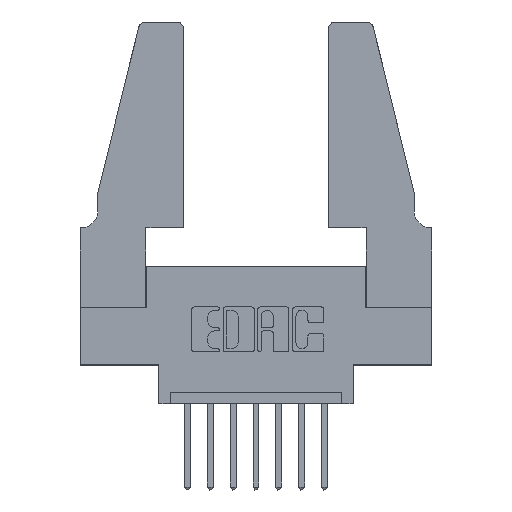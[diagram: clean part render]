
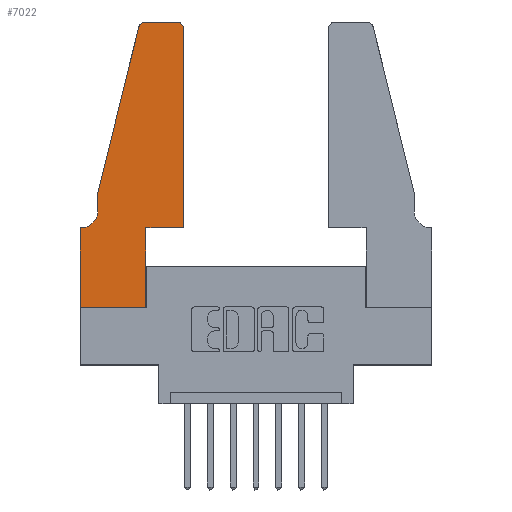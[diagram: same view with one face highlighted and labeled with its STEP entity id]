
A CAD part, top view. The second image highlights one B-rep face of the part: STEP entity #7022.
In plain terms, the highlighted planar face has unit normal (0, 0, 1).
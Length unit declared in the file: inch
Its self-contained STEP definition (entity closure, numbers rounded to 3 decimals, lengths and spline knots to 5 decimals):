
#166 = CARTESIAN_POINT ( 'NONE',  ( 0.0755, 0.42, 0.37 ) ) ;
#304 = LINE ( 'NONE', #4381, #5185 ) ;
#430 = CARTESIAN_POINT ( 'NONE',  ( 0.2865, 0.35, 0.37 ) ) ;
#513 = DIRECTION ( 'NONE',  ( 1., 0., 0. ) ) ;
#522 = LINE ( 'NONE', #9591, #1848 ) ;
#562 = CARTESIAN_POINT ( 'NONE',  ( 0.4505, 0.35, 0.37 ) ) ;
#626 = VECTOR ( 'NONE', #3883, 39.37008 ) ;
#668 = DIRECTION ( 'NONE',  ( 1., 0., 0. ) ) ;
#706 = VECTOR ( 'NONE', #9544, 39.37008 ) ;
#772 = CARTESIAN_POINT ( 'NONE',  ( 0.4205, 1.25, 0.37 ) ) ;
#1071 = VERTEX_POINT ( 'NONE', #3233 ) ;
#1128 = LINE ( 'NONE', #4679, #10800 ) ;
#1173 = CARTESIAN_POINT ( 'NONE',  ( 0.0755, 0.35, 0.37 ) ) ;
#1192 = VERTEX_POINT ( 'NONE', #3646 ) ;
#1230 = ORIENTED_EDGE ( 'NONE', *, *, #9600, .T. ) ;
#1241 = ORIENTED_EDGE ( 'NONE', *, *, #9522, .T. ) ;
#1252 = ORIENTED_EDGE ( 'NONE', *, *, #2379, .T. ) ;
#1300 = EDGE_CURVE ( 'NONE', #8471, #4289, #6045, .T. ) ;
#1409 = VERTEX_POINT ( 'NONE', #11845 ) ;
#1569 = EDGE_CURVE ( 'NONE', #11070, #6706, #1128, .T. ) ;
#1848 = VECTOR ( 'NONE', #3009, 39.37008 ) ;
#2005 = CARTESIAN_POINT ( 'NONE',  ( 0.0755, 0.5, 0.37 ) ) ;
#2217 = PLANE ( 'NONE',  #5233 ) ;
#2340 = CARTESIAN_POINT ( 'NONE',  ( 0., 0.35, 0.37 ) ) ;
#2379 = EDGE_CURVE ( 'NONE', #1192, #2687, #522, .T. ) ;
#2471 = DIRECTION ( 'NONE',  ( 0., 1., 0. ) ) ;
#2560 = EDGE_CURVE ( 'NONE', #1071, #8806, #4241, .T. ) ;
#2619 = DIRECTION ( 'NONE',  ( -0.239, -0.971, 0. ) ) ;
#2687 = VERTEX_POINT ( 'NONE', #9164 ) ;
#3009 = DIRECTION ( 'NONE',  ( 0., -1., 0. ) ) ;
#3233 = CARTESIAN_POINT ( 'NONE',  ( 0.4505, 1.22, 0.37 ) ) ;
#3252 = ORIENTED_EDGE ( 'NONE', *, *, #5866, .T. ) ;
#3311 = LINE ( 'NONE', #7150, #5851 ) ;
#3422 = ORIENTED_EDGE ( 'NONE', *, *, #2560, .T. ) ;
#3570 = DIRECTION ( 'NONE',  ( 0., 0., 1. ) ) ;
#3592 = LINE ( 'NONE', #1173, #626 ) ;
#3646 = CARTESIAN_POINT ( 'NONE',  ( 0., 0.35, 0.37 ) ) ;
#3883 = DIRECTION ( 'NONE',  ( -1., 0., 0. ) ) ;
#4055 = AXIS2_PLACEMENT_3D ( 'NONE', #4297, #11877, #513 ) ;
#4241 = CIRCLE ( 'NONE', #4984, 0.03 ) ;
#4289 = VERTEX_POINT ( 'NONE', #562 ) ;
#4297 = CARTESIAN_POINT ( 'NONE',  ( 0.284, 1.22, 0.37 ) ) ;
#4381 = CARTESIAN_POINT ( 'NONE',  ( 0., 0., 0.37 ) ) ;
#4478 = CARTESIAN_POINT ( 'NONE',  ( 0.0055, 0.35, 0.37 ) ) ;
#4501 = CIRCLE ( 'NONE', #4055, 0.03 ) ;
#4679 = CARTESIAN_POINT ( 'NONE',  ( 0.0755, 0.5, 0.37 ) ) ;
#4984 = AXIS2_PLACEMENT_3D ( 'NONE', #7502, #3570, #10185 ) ;
#5185 = VECTOR ( 'NONE', #9229, 39.37008 ) ;
#5233 = AXIS2_PLACEMENT_3D ( 'NONE', #2340, #7117, #668 ) ;
#5235 = CARTESIAN_POINT ( 'NONE',  ( 0.2605, 1.25, 0.37 ) ) ;
#5531 = VERTEX_POINT ( 'NONE', #4478 ) ;
#5595 = DIRECTION ( 'NONE',  ( 0., 0., -1. ) ) ;
#5612 = CARTESIAN_POINT ( 'NONE',  ( 0.2865, 0.35, 0.37 ) ) ;
#5851 = VECTOR ( 'NONE', #2471, 39.37008 ) ;
#5866 = EDGE_CURVE ( 'NONE', #4289, #1071, #3311, .T. ) ;
#6045 = LINE ( 'NONE', #9760, #6798 ) ;
#6062 = LINE ( 'NONE', #2005, #706 ) ;
#6106 = ORIENTED_EDGE ( 'NONE', *, *, #1569, .T. ) ;
#6109 = FACE_OUTER_BOUND ( 'NONE', #10574, .T. ) ;
#6207 = LINE ( 'NONE', #5235, #9185 ) ;
#6242 = EDGE_CURVE ( 'NONE', #5531, #1192, #3592, .T. ) ;
#6453 = EDGE_CURVE ( 'NONE', #1409, #11070, #4501, .T. ) ;
#6706 = VERTEX_POINT ( 'NONE', #6903 ) ;
#6798 = VECTOR ( 'NONE', #10586, 39.37008 ) ;
#6903 = CARTESIAN_POINT ( 'NONE',  ( 0.0755, 0.5, 0.37 ) ) ;
#7022 = ADVANCED_FACE ( 'NONE', ( #6109 ), #2217, .T. ) ;
#7117 = DIRECTION ( 'NONE',  ( 0., 0., 1. ) ) ;
#7150 = CARTESIAN_POINT ( 'NONE',  ( 0.4505, 0.35, 0.37 ) ) ;
#7208 = DIRECTION ( 'NONE',  ( -1., 0., 0. ) ) ;
#7502 = CARTESIAN_POINT ( 'NONE',  ( 0.4205, 1.22, 0.37 ) ) ;
#8159 = VECTOR ( 'NONE', #10027, 39.37008 ) ;
#8220 = ORIENTED_EDGE ( 'NONE', *, *, #1300, .T. ) ;
#8432 = CARTESIAN_POINT ( 'NONE',  ( 0.0055, 0.42, 0.37 ) ) ;
#8471 = VERTEX_POINT ( 'NONE', #5612 ) ;
#8630 = ORIENTED_EDGE ( 'NONE', *, *, #6453, .T. ) ;
#8806 = VERTEX_POINT ( 'NONE', #772 ) ;
#8972 = EDGE_CURVE ( 'NONE', #11306, #8471, #9056, .T. ) ;
#9056 = LINE ( 'NONE', #430, #8159 ) ;
#9095 = AXIS2_PLACEMENT_3D ( 'NONE', #8432, #5595, #10169 ) ;
#9146 = VERTEX_POINT ( 'NONE', #166 ) ;
#9164 = CARTESIAN_POINT ( 'NONE',  ( 0., 0., 0.37 ) ) ;
#9185 = VECTOR ( 'NONE', #7208, 39.37008 ) ;
#9229 = DIRECTION ( 'NONE',  ( 1., 0., 0. ) ) ;
#9327 = EDGE_CURVE ( 'NONE', #9146, #5531, #10827, .T. ) ;
#9522 = EDGE_CURVE ( 'NONE', #8806, #1409, #6207, .T. ) ;
#9528 = CARTESIAN_POINT ( 'NONE',  ( 0.25487, 1.22718, 0.37 ) ) ;
#9544 = DIRECTION ( 'NONE',  ( 0., -1., 0. ) ) ;
#9577 = ORIENTED_EDGE ( 'NONE', *, *, #8972, .T. ) ;
#9591 = CARTESIAN_POINT ( 'NONE',  ( 0., 0., 0.37 ) ) ;
#9600 = EDGE_CURVE ( 'NONE', #6706, #9146, #6062, .T. ) ;
#9760 = CARTESIAN_POINT ( 'NONE',  ( 0.4505, 0.35, 0.37 ) ) ;
#9893 = ORIENTED_EDGE ( 'NONE', *, *, #9327, .T. ) ;
#10012 = CARTESIAN_POINT ( 'NONE',  ( 0.2865, 0., 0.37 ) ) ;
#10027 = DIRECTION ( 'NONE',  ( 0., 1., 0. ) ) ;
#10169 = DIRECTION ( 'NONE',  ( -1., 0., 0. ) ) ;
#10185 = DIRECTION ( 'NONE',  ( 1., 0., 0. ) ) ;
#10574 = EDGE_LOOP ( 'NONE', ( #1241, #8630, #6106, #1230, #9893, #11031, #1252, #11193, #9577, #8220, #3252, #3422 ) ) ;
#10586 = DIRECTION ( 'NONE',  ( 1., 0., 0. ) ) ;
#10722 = EDGE_CURVE ( 'NONE', #2687, #11306, #304, .T. ) ;
#10800 = VECTOR ( 'NONE', #2619, 39.37008 ) ;
#10827 = CIRCLE ( 'NONE', #9095, 0.07 ) ;
#11031 = ORIENTED_EDGE ( 'NONE', *, *, #6242, .T. ) ;
#11070 = VERTEX_POINT ( 'NONE', #9528 ) ;
#11193 = ORIENTED_EDGE ( 'NONE', *, *, #10722, .T. ) ;
#11306 = VERTEX_POINT ( 'NONE', #10012 ) ;
#11845 = CARTESIAN_POINT ( 'NONE',  ( 0.284, 1.25, 0.37 ) ) ;
#11877 = DIRECTION ( 'NONE',  ( 0., 0., 1. ) ) ;
